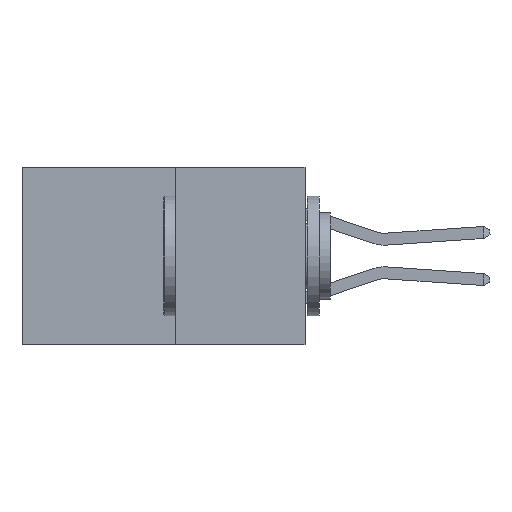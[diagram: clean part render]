
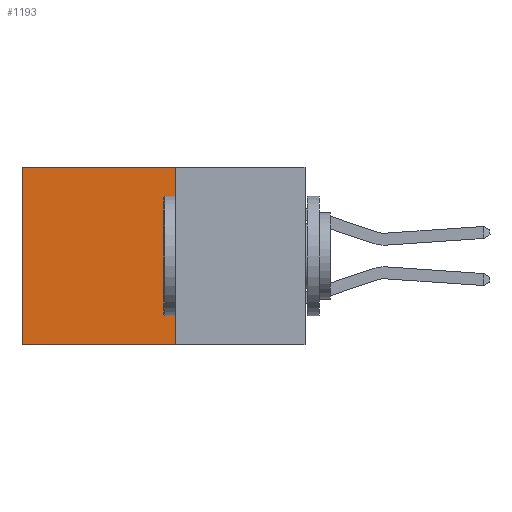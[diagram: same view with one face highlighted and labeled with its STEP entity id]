
A CAD part, left-side view. The second image highlights one B-rep face of the part: STEP entity #1193.
In plain terms, the highlighted planar face has unit normal (-1, 0, 0).
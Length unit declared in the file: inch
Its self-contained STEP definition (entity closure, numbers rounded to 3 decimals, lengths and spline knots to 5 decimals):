
#58 = CARTESIAN_POINT ( 'NONE',  ( 0.277, 0.27, 0. ) ) ;
#1193 = ADVANCED_FACE ( 'NONE', ( #5155 ), #5804, .F. ) ;
#1593 = CARTESIAN_POINT ( 'NONE',  ( 0.277, 0.59, -0.37 ) ) ;
#1855 = EDGE_LOOP ( 'NONE', ( #7284, #7170, #6535, #2441 ) ) ;
#1956 = VECTOR ( 'NONE', #3966, 39.37008 ) ;
#1983 = AXIS2_PLACEMENT_3D ( 'NONE', #3936, #7396, #8980 ) ;
#2441 = ORIENTED_EDGE ( 'NONE', *, *, #3081, .T. ) ;
#2688 = VECTOR ( 'NONE', #7131, 39.37008 ) ;
#2708 = VERTEX_POINT ( 'NONE', #4629 ) ;
#3081 = EDGE_CURVE ( 'NONE', #3601, #4940, #4576, .T. ) ;
#3094 = EDGE_CURVE ( 'NONE', #2708, #5612, #8372, .T. ) ;
#3601 = VERTEX_POINT ( 'NONE', #58 ) ;
#3936 = CARTESIAN_POINT ( 'NONE',  ( 0.277, 0.27, -0.37 ) ) ;
#3966 = DIRECTION ( 'NONE',  ( 0., 0., -1. ) ) ;
#4388 = EDGE_CURVE ( 'NONE', #4940, #5612, #8046, .T. ) ;
#4576 = LINE ( 'NONE', #7140, #2688 ) ;
#4629 = CARTESIAN_POINT ( 'NONE',  ( 0.277, 0.27, -0.37 ) ) ;
#4634 = CARTESIAN_POINT ( 'NONE',  ( 0.277, 0.27, -0.37 ) ) ;
#4940 = VERTEX_POINT ( 'NONE', #5318 ) ;
#5155 = FACE_OUTER_BOUND ( 'NONE', #1855, .T. ) ;
#5318 = CARTESIAN_POINT ( 'NONE',  ( 0.277, 0.59, 0. ) ) ;
#5612 = VERTEX_POINT ( 'NONE', #1593 ) ;
#5804 = PLANE ( 'NONE',  #1983 ) ;
#6303 = VECTOR ( 'NONE', #8589, 39.37008 ) ;
#6535 = ORIENTED_EDGE ( 'NONE', *, *, #7577, .F. ) ;
#6988 = CARTESIAN_POINT ( 'NONE',  ( 0.277, 0.27, -0.37 ) ) ;
#7005 = DIRECTION ( 'NONE',  ( 0., 1., 0. ) ) ;
#7131 = DIRECTION ( 'NONE',  ( 0., 1., 0. ) ) ;
#7140 = CARTESIAN_POINT ( 'NONE',  ( 0.277, 0.27, 0. ) ) ;
#7170 = ORIENTED_EDGE ( 'NONE', *, *, #3094, .F. ) ;
#7284 = ORIENTED_EDGE ( 'NONE', *, *, #4388, .T. ) ;
#7396 = DIRECTION ( 'NONE',  ( 1., 0., 0. ) ) ;
#7545 = LINE ( 'NONE', #4634, #1956 ) ;
#7577 = EDGE_CURVE ( 'NONE', #3601, #2708, #7545, .T. ) ;
#7964 = VECTOR ( 'NONE', #7005, 39.37008 ) ;
#8046 = LINE ( 'NONE', #8615, #6303 ) ;
#8372 = LINE ( 'NONE', #6988, #7964 ) ;
#8589 = DIRECTION ( 'NONE',  ( 0., 0., -1. ) ) ;
#8615 = CARTESIAN_POINT ( 'NONE',  ( 0.277, 0.59, -0.37 ) ) ;
#8980 = DIRECTION ( 'NONE',  ( 0., 0., -1. ) ) ;
